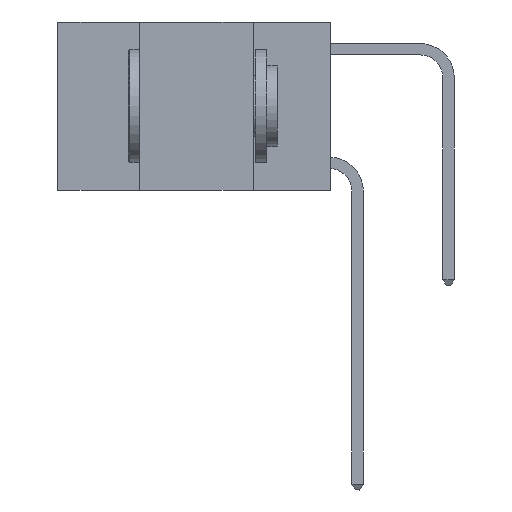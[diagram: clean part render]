
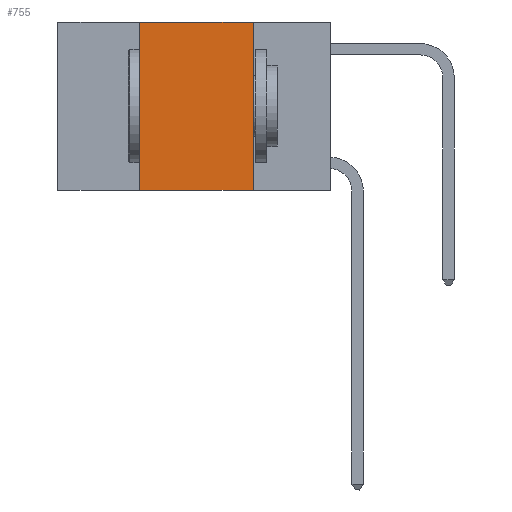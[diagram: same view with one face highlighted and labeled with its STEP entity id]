
A CAD part, left-side view. The second image highlights one B-rep face of the part: STEP entity #755.
In plain terms, the highlighted planar face has unit normal (-1, 0, 0).
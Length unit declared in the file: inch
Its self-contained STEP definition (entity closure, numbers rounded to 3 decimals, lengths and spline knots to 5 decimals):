
#755 = ADVANCED_FACE ( 'NONE', ( #2857 ), #20637, .F. ) ;
#1198 = CARTESIAN_POINT ( 'NONE',  ( 0., 0.6, 0. ) ) ;
#1599 = VECTOR ( 'NONE', #24359, 39.37008 ) ;
#1987 = VERTEX_POINT ( 'NONE', #14161 ) ;
#2857 = FACE_OUTER_BOUND ( 'NONE', #21306, .T. ) ;
#3008 = CARTESIAN_POINT ( 'NONE',  ( 0., 0.42, 0. ) ) ;
#3258 = DIRECTION ( 'NONE',  ( 1., 0., 0. ) ) ;
#3295 = LINE ( 'NONE', #15057, #13270 ) ;
#4356 = EDGE_CURVE ( 'NONE', #11155, #20852, #23904, .T. ) ;
#5280 = EDGE_CURVE ( 'NONE', #5632, #20852, #3295, .T. ) ;
#5632 = VERTEX_POINT ( 'NONE', #25062 ) ;
#6533 = CARTESIAN_POINT ( 'NONE',  ( 0., 0.17, 0. ) ) ;
#8193 = DIRECTION ( 'NONE',  ( 0., -1., 0. ) ) ;
#8677 = AXIS2_PLACEMENT_3D ( 'NONE', #1198, #3258, #22679 ) ;
#9177 = VECTOR ( 'NONE', #8193, 39.37008 ) ;
#9933 = EDGE_CURVE ( 'NONE', #5632, #1987, #24598, .T. ) ;
#9978 = CARTESIAN_POINT ( 'NONE',  ( 0., 0.6, 0. ) ) ;
#11155 = VERTEX_POINT ( 'NONE', #22088 ) ;
#11348 = ORIENTED_EDGE ( 'NONE', *, *, #18528, .F. ) ;
#12280 = DIRECTION ( 'NONE',  ( 0., 0., -1. ) ) ;
#13270 = VECTOR ( 'NONE', #22847, 39.37008 ) ;
#14161 = CARTESIAN_POINT ( 'NONE',  ( 0., 0.42, 0. ) ) ;
#15057 = CARTESIAN_POINT ( 'NONE',  ( 0., 0.6, -0.37 ) ) ;
#15738 = VECTOR ( 'NONE', #12280, 39.37008 ) ;
#18388 = CARTESIAN_POINT ( 'NONE',  ( 0., 0.17, -0.37 ) ) ;
#18528 = EDGE_CURVE ( 'NONE', #1987, #11155, #23754, .T. ) ;
#19871 = ORIENTED_EDGE ( 'NONE', *, *, #5280, .T. ) ;
#20228 = ORIENTED_EDGE ( 'NONE', *, *, #9933, .F. ) ;
#20637 = PLANE ( 'NONE',  #8677 ) ;
#20852 = VERTEX_POINT ( 'NONE', #18388 ) ;
#21306 = EDGE_LOOP ( 'NONE', ( #24076, #11348, #20228, #19871 ) ) ;
#22088 = CARTESIAN_POINT ( 'NONE',  ( 0., 0.17, 0. ) ) ;
#22679 = DIRECTION ( 'NONE',  ( 0., 0., -1. ) ) ;
#22847 = DIRECTION ( 'NONE',  ( 0., -1., 0. ) ) ;
#23754 = LINE ( 'NONE', #9978, #9177 ) ;
#23904 = LINE ( 'NONE', #6533, #15738 ) ;
#24076 = ORIENTED_EDGE ( 'NONE', *, *, #4356, .F. ) ;
#24359 = DIRECTION ( 'NONE',  ( 0., 0., 1. ) ) ;
#24598 = LINE ( 'NONE', #3008, #1599 ) ;
#25062 = CARTESIAN_POINT ( 'NONE',  ( 0., 0.42, -0.37 ) ) ;
